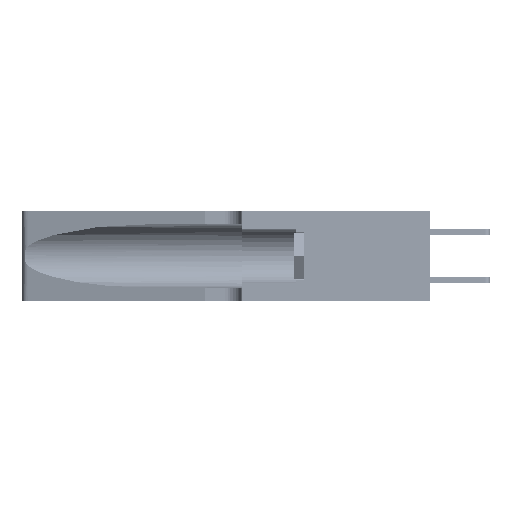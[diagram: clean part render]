
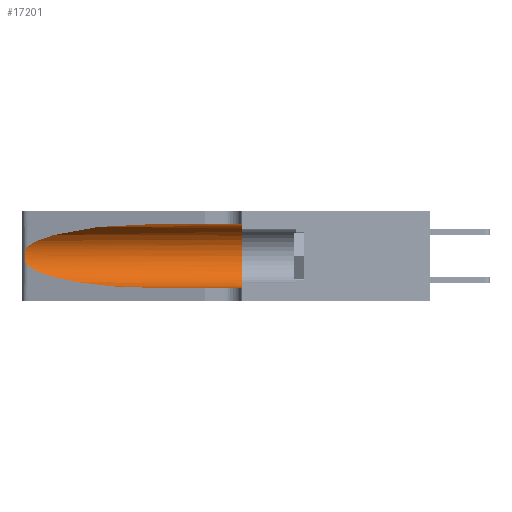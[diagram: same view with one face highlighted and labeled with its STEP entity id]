
A CAD part, left-side view. The second image highlights one B-rep face of the part: STEP entity #17201.
In plain terms, the highlighted cylindrical face has radius 3.308 mm (diameter 6.617 mm), a partial arc.
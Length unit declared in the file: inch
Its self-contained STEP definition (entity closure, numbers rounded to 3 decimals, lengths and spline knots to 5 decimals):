
#400 = B_SPLINE_CURVE_WITH_KNOTS ( 'NONE', 3,
 ( #24466, #27795, #11441, #5042, #4427, #37047, #27931, #31225, #17429, #8326, #20708, #30625, #10997, #33911 ),
 .UNSPECIFIED., .F., .F.,
 ( 4, 2, 2, 2, 2, 2, 4 ),
 ( 0., 0.00027, 0.00053, 0.00107, 0.0016, 0.00187, 0.00214 ),
 .UNSPECIFIED. ) ;
#1028 = CARTESIAN_POINT ( 'NONE',  ( 0.25487, 1.22718, 0.22369 ) ) ;
#1034 = VERTEX_POINT ( 'NONE', #6970 ) ;
#1076 = VERTEX_POINT ( 'NONE', #20090 ) ;
#1764 = DIRECTION ( 'NONE',  ( 0., 1., 0. ) ) ;
#1779 = CARTESIAN_POINT ( 'NONE',  ( 0.1305, 0.72297, 0.05475 ) ) ;
#2152 = CARTESIAN_POINT ( 'NONE',  ( 0.25487, 1.22718, 0.22369 ) ) ;
#4427 = CARTESIAN_POINT ( 'NONE',  ( 0.25854, 1.2359, 0.20912 ) ) ;
#5042 = CARTESIAN_POINT ( 'NONE',  ( 0.25787, 1.23484, 0.2124 ) ) ;
#6970 = CARTESIAN_POINT ( 'NONE',  ( 0.25487, 1.22718, 0.14631 ) ) ;
#7374 = CARTESIAN_POINT ( 'NONE',  ( 0.1305, 0.72297, 0.05475 ) ) ;
#7781 = EDGE_CURVE ( 'NONE', #1034, #40661, #32966, .T. ) ;
#8326 = CARTESIAN_POINT ( 'NONE',  ( 0.25856, 1.23593, 0.16098 ) ) ;
#8532 = VERTEX_POINT ( 'NONE', #2152 ) ;
#9961 = ORIENTED_EDGE ( 'NONE', *, *, #14065, .T. ) ;
#10997 = CARTESIAN_POINT ( 'NONE',  ( 0.25555, 1.22993, 0.14849 ) ) ;
#11013 = EDGE_CURVE ( 'NONE', #1076, #31266, #19651, .T. ) ;
#11441 = CARTESIAN_POINT ( 'NONE',  ( 0.25639, 1.23184, 0.21858 ) ) ;
#11501 = VECTOR ( 'NONE', #18501, 39.37008 ) ;
#11923 = CARTESIAN_POINT ( 'NONE',  ( 0.25487, 1.22718, 0.14631 ) ) ;
#11987 = CYLINDRICAL_SURFACE ( 'NONE', #23171, 0.13025 ) ;
#12361 = ORIENTED_EDGE ( 'NONE', *, *, #16085, .T. ) ;
#12509 = EDGE_CURVE ( 'NONE', #31266, #36446, #14422, .T. ) ;
#12536 =( BOUNDED_CURVE ( )  B_SPLINE_CURVE ( 3, ( #33541, #13930, #17214, #1028 ),
 .UNSPECIFIED., .F., .F. ) 
 B_SPLINE_CURVE_WITH_KNOTS ( ( 4, 4 ),
 ( 1.5708, 2.84003 ),
 .UNSPECIFIED. ) 
 CURVE ( )  GEOMETRIC_REPRESENTATION_ITEM ( )  RATIONAL_B_SPLINE_CURVE ( ( 1., 0.87, 0.87, 1. ) ) 
 REPRESENTATION_ITEM ( '' )  );
#13930 = CARTESIAN_POINT ( 'NONE',  ( 0.18966, 0.96281, 0.31525 ) ) ;
#14063 = CARTESIAN_POINT ( 'NONE',  ( 0.1305, 1.61858, 0.185 ) ) ;
#14065 = EDGE_CURVE ( 'NONE', #8532, #1034, #400, .T. ) ;
#14422 = CIRCLE ( 'NONE', #15952, 0.13025 ) ;
#15952 = AXIS2_PLACEMENT_3D ( 'NONE', #18216, #1764, #29121 ) ;
#16085 = EDGE_CURVE ( 'NONE', #40661, #36446, #32587, .T. ) ;
#17201 = ADVANCED_FACE ( 'NONE', ( #19652 ), #11987, .F. ) ;
#17214 = CARTESIAN_POINT ( 'NONE',  ( 0.2373, 1.15595, 0.28018 ) ) ;
#17429 = CARTESIAN_POINT ( 'NONE',  ( 0.26017, 1.23833, 0.17102 ) ) ;
#17954 = CARTESIAN_POINT ( 'NONE',  ( 0.2373, 1.15595, 0.08982 ) ) ;
#18216 = CARTESIAN_POINT ( 'NONE',  ( 0.1305, 0.35, 0.185 ) ) ;
#18501 = DIRECTION ( 'NONE',  ( 0., -1., 0. ) ) ;
#18519 = CARTESIAN_POINT ( 'NONE',  ( 0.1305, 1.61858, 0.05475 ) ) ;
#18638 = CARTESIAN_POINT ( 'NONE',  ( 0.1305, 1.61858, 0.31525 ) ) ;
#19156 = ORIENTED_EDGE ( 'NONE', *, *, #7781, .T. ) ;
#19651 = LINE ( 'NONE', #18638, #11501 ) ;
#19652 = FACE_OUTER_BOUND ( 'NONE', #19712, .T. ) ;
#19712 = EDGE_LOOP ( 'NONE', ( #25303, #9961, #19156, #12361, #32892, #20274 ) ) ;
#20090 = CARTESIAN_POINT ( 'NONE',  ( 0.1305, 0.72297, 0.31525 ) ) ;
#20274 = ORIENTED_EDGE ( 'NONE', *, *, #11013, .F. ) ;
#20708 = CARTESIAN_POINT ( 'NONE',  ( 0.25789, 1.23486, 0.15765 ) ) ;
#21834 = VECTOR ( 'NONE', #41007, 39.37008 ) ;
#23171 = AXIS2_PLACEMENT_3D ( 'NONE', #14063, #36976, #30859 ) ;
#24466 = CARTESIAN_POINT ( 'NONE',  ( 0.25487, 1.22718, 0.22369 ) ) ;
#25303 = ORIENTED_EDGE ( 'NONE', *, *, #35017, .T. ) ;
#27795 = CARTESIAN_POINT ( 'NONE',  ( 0.25555, 1.22994, 0.2215 ) ) ;
#27931 = CARTESIAN_POINT ( 'NONE',  ( 0.26075, 1.23896, 0.19203 ) ) ;
#29121 = DIRECTION ( 'NONE',  ( 0., 0., 1. ) ) ;
#30625 = CARTESIAN_POINT ( 'NONE',  ( 0.25639, 1.23186, 0.15144 ) ) ;
#30859 = DIRECTION ( 'NONE',  ( 0., 0., -1. ) ) ;
#31225 = CARTESIAN_POINT ( 'NONE',  ( 0.26075, 1.23896, 0.178 ) ) ;
#31266 = VERTEX_POINT ( 'NONE', #37243 ) ;
#32587 = LINE ( 'NONE', #18519, #21834 ) ;
#32892 = ORIENTED_EDGE ( 'NONE', *, *, #12509, .F. ) ;
#32966 =( BOUNDED_CURVE ( )  B_SPLINE_CURVE ( 3, ( #11923, #17954, #34989, #1779 ),
 .UNSPECIFIED., .F., .F. ) 
 B_SPLINE_CURVE_WITH_KNOTS ( ( 4, 4 ),
 ( 3.44316, 4.71239 ),
 .UNSPECIFIED. ) 
 CURVE ( )  GEOMETRIC_REPRESENTATION_ITEM ( )  RATIONAL_B_SPLINE_CURVE ( ( 1., 0.87, 0.87, 1. ) ) 
 REPRESENTATION_ITEM ( '' )  );
#33541 = CARTESIAN_POINT ( 'NONE',  ( 0.1305, 0.72297, 0.31525 ) ) ;
#33795 = CARTESIAN_POINT ( 'NONE',  ( 0.1305, 0.35, 0.05475 ) ) ;
#33911 = CARTESIAN_POINT ( 'NONE',  ( 0.25487, 1.22718, 0.14631 ) ) ;
#34989 = CARTESIAN_POINT ( 'NONE',  ( 0.18966, 0.96281, 0.05475 ) ) ;
#35017 = EDGE_CURVE ( 'NONE', #1076, #8532, #12536, .T. ) ;
#36446 = VERTEX_POINT ( 'NONE', #33795 ) ;
#36976 = DIRECTION ( 'NONE',  ( 0., -1., 0. ) ) ;
#37047 = CARTESIAN_POINT ( 'NONE',  ( 0.26018, 1.23835, 0.19895 ) ) ;
#37243 = CARTESIAN_POINT ( 'NONE',  ( 0.1305, 0.35, 0.31525 ) ) ;
#40661 = VERTEX_POINT ( 'NONE', #7374 ) ;
#41007 = DIRECTION ( 'NONE',  ( 0., -1., 0. ) ) ;
